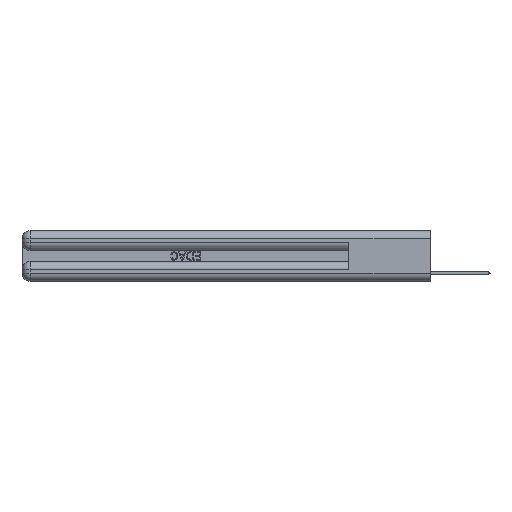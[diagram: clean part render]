
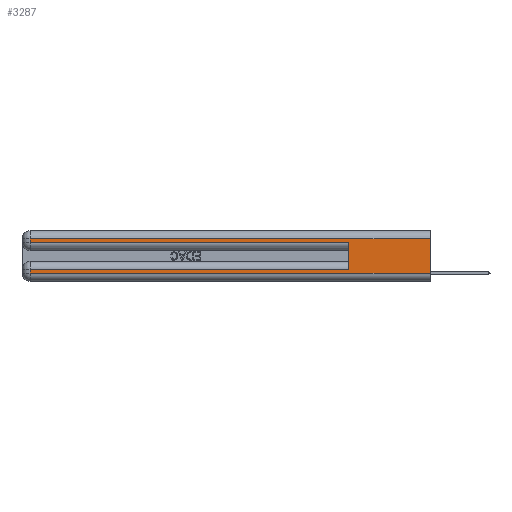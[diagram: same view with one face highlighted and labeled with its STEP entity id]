
A CAD part, left-side view. The second image highlights one B-rep face of the part: STEP entity #3287.
In plain terms, the highlighted planar face has unit normal (-1, 0, 0).
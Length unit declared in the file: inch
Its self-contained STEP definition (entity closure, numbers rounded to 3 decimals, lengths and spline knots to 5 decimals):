
#1029 = LINE ( 'NONE', #27405, #13135 ) ;
#1149 = EDGE_CURVE ( 'NONE', #9564, #14840, #1029, .T. ) ;
#1972 = EDGE_CURVE ( 'NONE', #13393, #9564, #26126, .T. ) ;
#2187 = CARTESIAN_POINT ( 'NONE',  ( 0., 2.94, 0.285 ) ) ;
#2747 = VECTOR ( 'NONE', #12849, 39.37008 ) ;
#2844 = VERTEX_POINT ( 'NONE', #12740 ) ;
#2865 = EDGE_CURVE ( 'NONE', #14840, #2844, #5879, .T. ) ;
#3287 = ADVANCED_FACE ( 'NONE', ( #19866 ), #16066, .F. ) ;
#3433 = VERTEX_POINT ( 'NONE', #27177 ) ;
#3970 = CARTESIAN_POINT ( 'NONE',  ( 0., 0.6, 0.145 ) ) ;
#5318 = CARTESIAN_POINT ( 'NONE',  ( 0., 2.94, 0.37 ) ) ;
#5879 = LINE ( 'NONE', #12894, #28471 ) ;
#5895 = CARTESIAN_POINT ( 'NONE',  ( 0., 0.6, 0.285 ) ) ;
#6634 = EDGE_CURVE ( 'NONE', #13393, #22898, #26124, .T. ) ;
#6838 = VECTOR ( 'NONE', #18101, 39.37008 ) ;
#7052 = ORIENTED_EDGE ( 'NONE', *, *, #12235, .F. ) ;
#7107 = DIRECTION ( 'NONE',  ( 0., 0., -1. ) ) ;
#7498 = CARTESIAN_POINT ( 'NONE',  ( 0., 2.94, 0.06 ) ) ;
#7970 = DIRECTION ( 'NONE',  ( 0., -1., 0. ) ) ;
#8557 = DIRECTION ( 'NONE',  ( 0., 0., -1. ) ) ;
#8791 = DIRECTION ( 'NONE',  ( 0., 0., -1. ) ) ;
#9564 = VERTEX_POINT ( 'NONE', #26338 ) ;
#10489 = AXIS2_PLACEMENT_3D ( 'NONE', #26539, #15518, #8791 ) ;
#11530 = VECTOR ( 'NONE', #7970, 39.37008 ) ;
#12208 = EDGE_LOOP ( 'NONE', ( #7052, #16225, #22604, #27473, #15042, #19862, #14878, #27845 ) ) ;
#12235 = EDGE_CURVE ( 'NONE', #3433, #2844, #13367, .T. ) ;
#12740 = CARTESIAN_POINT ( 'NONE',  ( 0., 0., 0.06 ) ) ;
#12849 = DIRECTION ( 'NONE',  ( 0., 0., 1. ) ) ;
#12894 = CARTESIAN_POINT ( 'NONE',  ( 0., 0., 0.06 ) ) ;
#13135 = VECTOR ( 'NONE', #23337, 39.37008 ) ;
#13298 = DIRECTION ( 'NONE',  ( 0., 1., 0. ) ) ;
#13367 = LINE ( 'NONE', #28501, #28269 ) ;
#13393 = VERTEX_POINT ( 'NONE', #19492 ) ;
#13571 = LINE ( 'NONE', #17817, #6838 ) ;
#14840 = VERTEX_POINT ( 'NONE', #7498 ) ;
#14878 = ORIENTED_EDGE ( 'NONE', *, *, #1149, .T. ) ;
#15042 = ORIENTED_EDGE ( 'NONE', *, *, #6634, .F. ) ;
#15518 = DIRECTION ( 'NONE',  ( 1., 0., 0. ) ) ;
#15780 = CARTESIAN_POINT ( 'NONE',  ( 0., 2.94, 0.31 ) ) ;
#16066 = PLANE ( 'NONE',  #10489 ) ;
#16225 = ORIENTED_EDGE ( 'NONE', *, *, #16301, .T. ) ;
#16301 = EDGE_CURVE ( 'NONE', #3433, #17328, #13571, .T. ) ;
#16676 = EDGE_CURVE ( 'NONE', #27036, #22898, #17320, .T. ) ;
#17320 = LINE ( 'NONE', #18898, #11530 ) ;
#17328 = VERTEX_POINT ( 'NONE', #15780 ) ;
#17817 = CARTESIAN_POINT ( 'NONE',  ( 0., 0., 0.31 ) ) ;
#18101 = DIRECTION ( 'NONE',  ( 0., 1., 0. ) ) ;
#18898 = CARTESIAN_POINT ( 'NONE',  ( 0., 0., 0.285 ) ) ;
#19492 = CARTESIAN_POINT ( 'NONE',  ( 0., 0.6, 0.085 ) ) ;
#19862 = ORIENTED_EDGE ( 'NONE', *, *, #1972, .T. ) ;
#19866 = FACE_OUTER_BOUND ( 'NONE', #12208, .T. ) ;
#20669 = VECTOR ( 'NONE', #7107, 39.37008 ) ;
#21769 = DIRECTION ( 'NONE',  ( 0., -1., 0. ) ) ;
#22604 = ORIENTED_EDGE ( 'NONE', *, *, #26025, .T. ) ;
#22898 = VERTEX_POINT ( 'NONE', #5895 ) ;
#23337 = DIRECTION ( 'NONE',  ( 0., 0., -1. ) ) ;
#25195 = VECTOR ( 'NONE', #13298, 39.37008 ) ;
#25319 = LINE ( 'NONE', #5318, #20669 ) ;
#26025 = EDGE_CURVE ( 'NONE', #17328, #27036, #25319, .T. ) ;
#26124 = LINE ( 'NONE', #3970, #2747 ) ;
#26126 = LINE ( 'NONE', #28436, #25195 ) ;
#26338 = CARTESIAN_POINT ( 'NONE',  ( 0., 2.94, 0.085 ) ) ;
#26539 = CARTESIAN_POINT ( 'NONE',  ( 0., 0., 0.37 ) ) ;
#27036 = VERTEX_POINT ( 'NONE', #2187 ) ;
#27177 = CARTESIAN_POINT ( 'NONE',  ( 0., 0., 0.31 ) ) ;
#27405 = CARTESIAN_POINT ( 'NONE',  ( 0., 2.94, 0.37 ) ) ;
#27473 = ORIENTED_EDGE ( 'NONE', *, *, #16676, .T. ) ;
#27845 = ORIENTED_EDGE ( 'NONE', *, *, #2865, .T. ) ;
#28269 = VECTOR ( 'NONE', #8557, 39.37008 ) ;
#28436 = CARTESIAN_POINT ( 'NONE',  ( 0., 0., 0.085 ) ) ;
#28471 = VECTOR ( 'NONE', #21769, 39.37008 ) ;
#28501 = CARTESIAN_POINT ( 'NONE',  ( 0., 0., 0.37 ) ) ;
